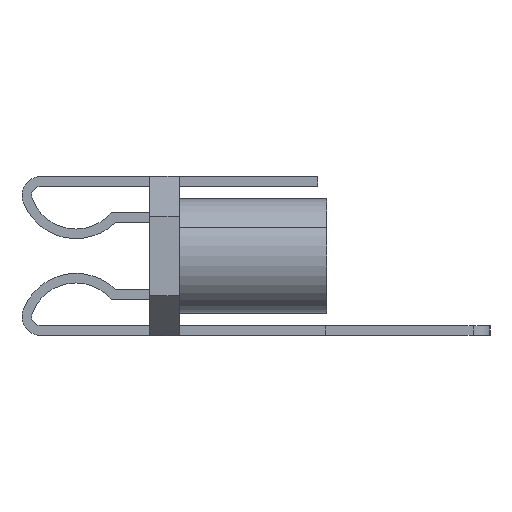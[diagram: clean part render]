
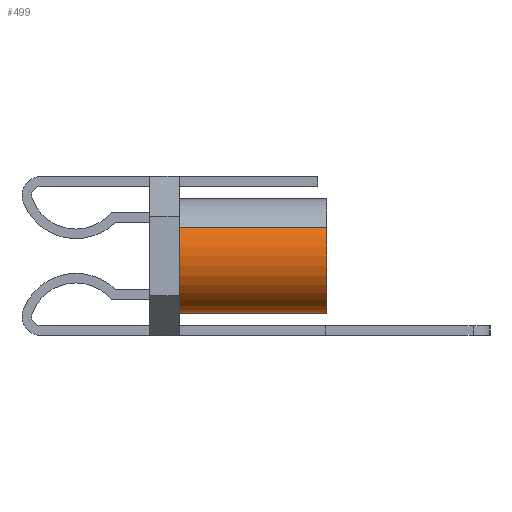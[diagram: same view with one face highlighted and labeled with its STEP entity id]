
A CAD part, left-side view. The second image highlights one B-rep face of the part: STEP entity #499.
In plain terms, the highlighted cylindrical face has radius 1.968 mm (diameter 3.937 mm), a partial arc.
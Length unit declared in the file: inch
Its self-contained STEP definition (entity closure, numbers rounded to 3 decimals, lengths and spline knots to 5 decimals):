
#499 = ADVANCED_FACE ( 'NONE', ( #5133 ), #7554, .T. ) ;
#2058 = LINE ( 'NONE', #5780, #9949 ) ;
#2545 = AXIS2_PLACEMENT_3D ( 'NONE', #12028, #11736, #11717 ) ;
#3134 = VERTEX_POINT ( 'NONE', #7779 ) ;
#3239 = EDGE_CURVE ( 'NONE', #4695, #5993, #8247, .T. ) ;
#4695 = VERTEX_POINT ( 'NONE', #11349 ) ;
#4758 = DIRECTION ( 'NONE',  ( 0., -1., 0. ) ) ;
#4897 = ORIENTED_EDGE ( 'NONE', *, *, #3239, .F. ) ;
#5133 = FACE_OUTER_BOUND ( 'NONE', #5871, .T. ) ;
#5229 = ORIENTED_EDGE ( 'NONE', *, *, #7309, .T. ) ;
#5243 = ORIENTED_EDGE ( 'NONE', *, *, #7312, .T. ) ;
#5287 = ORIENTED_EDGE ( 'NONE', *, *, #7293, .F. ) ;
#5780 = CARTESIAN_POINT ( 'NONE',  ( 0., 0.24, -0.0775 ) ) ;
#5829 = DIRECTION ( 'NONE',  ( 0., 1., 0. ) ) ;
#5871 = EDGE_LOOP ( 'NONE', ( #4897, #5229, #5243, #5287 ) ) ;
#5993 = VERTEX_POINT ( 'NONE', #12411 ) ;
#6824 = DIRECTION ( 'NONE',  ( 0., -1., 0. ) ) ;
#7293 = EDGE_CURVE ( 'NONE', #5993, #3134, #2058, .T. ) ;
#7309 = EDGE_CURVE ( 'NONE', #4695, #8844, #7677, .T. ) ;
#7312 = EDGE_CURVE ( 'NONE', #8844, #3134, #7368, .T. ) ;
#7368 = CIRCLE ( 'NONE', #11823, 0.0775 ) ;
#7554 = CYLINDRICAL_SURFACE ( 'NONE', #8163, 0.0775 ) ;
#7677 = LINE ( 'NONE', #11452, #12452 ) ;
#7779 = CARTESIAN_POINT ( 'NONE',  ( 0., 0.04, -0.0775 ) ) ;
#7815 = DIRECTION ( 'NONE',  ( 0., -1., 0. ) ) ;
#7977 = DIRECTION ( 'NONE',  ( 0., 0., -1. ) ) ;
#8163 = AXIS2_PLACEMENT_3D ( 'NONE', #9100, #4758, #7977 ) ;
#8247 = CIRCLE ( 'NONE', #2545, 0.0775 ) ;
#8844 = VERTEX_POINT ( 'NONE', #9426 ) ;
#9100 = CARTESIAN_POINT ( 'NONE',  ( 0., 0.24, 0. ) ) ;
#9426 = CARTESIAN_POINT ( 'NONE',  ( 0., 0.04, 0.0775 ) ) ;
#9949 = VECTOR ( 'NONE', #7815, 39.37008 ) ;
#11349 = CARTESIAN_POINT ( 'NONE',  ( 0., 0.24, 0.0775 ) ) ;
#11452 = CARTESIAN_POINT ( 'NONE',  ( 0., 0.24, 0.0775 ) ) ;
#11481 = CARTESIAN_POINT ( 'NONE',  ( 0., 0.04, 0. ) ) ;
#11717 = DIRECTION ( 'NONE',  ( 0., 0., 1. ) ) ;
#11736 = DIRECTION ( 'NONE',  ( 0., 1., 0. ) ) ;
#11823 = AXIS2_PLACEMENT_3D ( 'NONE', #11481, #5829, #12322 ) ;
#12028 = CARTESIAN_POINT ( 'NONE',  ( 0., 0.24, 0. ) ) ;
#12322 = DIRECTION ( 'NONE',  ( 0., 0., 1. ) ) ;
#12411 = CARTESIAN_POINT ( 'NONE',  ( 0., 0.24, -0.0775 ) ) ;
#12452 = VECTOR ( 'NONE', #6824, 39.37008 ) ;
